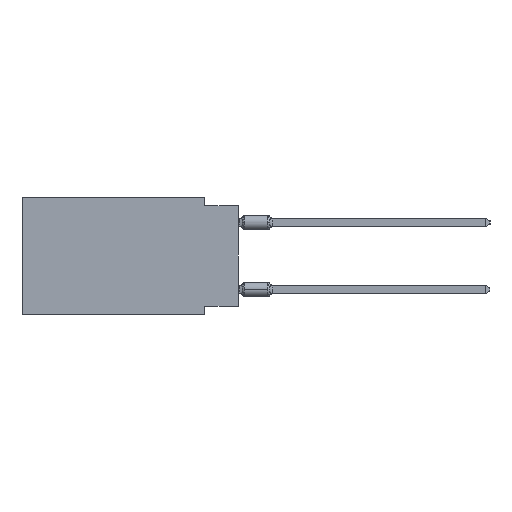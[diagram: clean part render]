
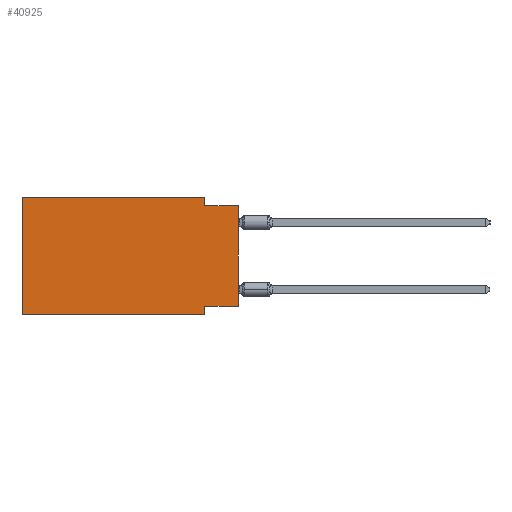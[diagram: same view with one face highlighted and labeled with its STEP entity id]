
A CAD part, left-side view. The second image highlights one B-rep face of the part: STEP entity #40925.
In plain terms, the highlighted planar face has unit normal (-1, 0, 0).
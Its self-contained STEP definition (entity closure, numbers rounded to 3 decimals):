
#448 = CARTESIAN_POINT ( 'NONE',  ( 0., 2.54, 0. ) ) ;
#1069 = VERTEX_POINT ( 'NONE', #16602 ) ;
#1219 = FACE_OUTER_BOUND ( 'NONE', #28514, .T. ) ;
#2025 = ORIENTED_EDGE ( 'NONE', *, *, #58208, .F. ) ;
#2263 = VECTOR ( 'NONE', #45250, 1000. ) ;
#3773 = CARTESIAN_POINT ( 'NONE',  ( 0., 2.54, -8.255 ) ) ;
#6072 = DIRECTION ( 'NONE',  ( 0., 0., -1. ) ) ;
#8190 = EDGE_CURVE ( 'NONE', #1069, #47045, #20040, .T. ) ;
#9418 = ORIENTED_EDGE ( 'NONE', *, *, #8190, .T. ) ;
#11039 = DIRECTION ( 'NONE',  ( 0., -1., 0. ) ) ;
#12231 = DIRECTION ( 'NONE',  ( 0., 1., 0. ) ) ;
#12298 = VERTEX_POINT ( 'NONE', #34679 ) ;
#12515 = VECTOR ( 'NONE', #12231, 1000. ) ;
#12544 = DIRECTION ( 'NONE',  ( 0., -1., 0. ) ) ;
#15291 = CARTESIAN_POINT ( 'NONE',  ( 0., 16.383, -8.89 ) ) ;
#15365 = VERTEX_POINT ( 'NONE', #53894 ) ;
#15708 = LINE ( 'NONE', #55323, #2263 ) ;
#16602 = CARTESIAN_POINT ( 'NONE',  ( 0., 0., -8.255 ) ) ;
#17701 = EDGE_CURVE ( 'NONE', #12298, #33344, #37183, .T. ) ;
#17742 = LINE ( 'NONE', #42714, #12515 ) ;
#17853 = VECTOR ( 'NONE', #39178, 1000. ) ;
#19060 = LINE ( 'NONE', #32686, #24188 ) ;
#19545 = VECTOR ( 'NONE', #12544, 1000. ) ;
#19724 = VERTEX_POINT ( 'NONE', #61601 ) ;
#20040 = LINE ( 'NONE', #44053, #17853 ) ;
#21690 = ORIENTED_EDGE ( 'NONE', *, *, #17701, .F. ) ;
#21887 = VERTEX_POINT ( 'NONE', #61754 ) ;
#24188 = VECTOR ( 'NONE', #29116, 1000. ) ;
#24577 = ORIENTED_EDGE ( 'NONE', *, *, #39522, .F. ) ;
#26257 = CARTESIAN_POINT ( 'NONE',  ( 0., 0., -0.635 ) ) ;
#27260 = ORIENTED_EDGE ( 'NONE', *, *, #46642, .F. ) ;
#28514 = EDGE_LOOP ( 'NONE', ( #9418, #2025, #44490, #21690, #63071, #38882, #27260, #24577 ) ) ;
#28870 = VECTOR ( 'NONE', #45242, 1000. ) ;
#29116 = DIRECTION ( 'NONE',  ( 0., -1., 0. ) ) ;
#31459 = EDGE_CURVE ( 'NONE', #21887, #15365, #49996, .T. ) ;
#32686 = CARTESIAN_POINT ( 'NONE',  ( 0., 0., -0.635 ) ) ;
#33344 = VERTEX_POINT ( 'NONE', #39706 ) ;
#34329 = DIRECTION ( 'NONE',  ( 1., 0., 0. ) ) ;
#34679 = CARTESIAN_POINT ( 'NONE',  ( 0., 16.383, 0. ) ) ;
#36195 = VERTEX_POINT ( 'NONE', #3773 ) ;
#37183 = LINE ( 'NONE', #57004, #19545 ) ;
#38882 = ORIENTED_EDGE ( 'NONE', *, *, #31459, .T. ) ;
#39178 = DIRECTION ( 'NONE',  ( 0., 0., 1. ) ) ;
#39522 = EDGE_CURVE ( 'NONE', #1069, #36195, #17742, .T. ) ;
#39706 = CARTESIAN_POINT ( 'NONE',  ( 0., 2.54, 0. ) ) ;
#39910 = VECTOR ( 'NONE', #11039, 1000. ) ;
#40925 = ADVANCED_FACE ( 'NONE', ( #1219 ), #50556, .F. ) ;
#41495 = VECTOR ( 'NONE', #61771, 1000. ) ;
#42714 = CARTESIAN_POINT ( 'NONE',  ( 0., 0., -8.255 ) ) ;
#44053 = CARTESIAN_POINT ( 'NONE',  ( 0., 0., 0. ) ) ;
#44490 = ORIENTED_EDGE ( 'NONE', *, *, #57133, .F. ) ;
#45242 = DIRECTION ( 'NONE',  ( 0., 0., -1. ) ) ;
#45250 = DIRECTION ( 'NONE',  ( 0., 0., 1. ) ) ;
#46642 = EDGE_CURVE ( 'NONE', #36195, #15365, #50112, .T. ) ;
#47002 = AXIS2_PLACEMENT_3D ( 'NONE', #59338, #34329, #6072 ) ;
#47045 = VERTEX_POINT ( 'NONE', #26257 ) ;
#49717 = EDGE_CURVE ( 'NONE', #21887, #12298, #15708, .T. ) ;
#49996 = LINE ( 'NONE', #15291, #39910 ) ;
#50112 = LINE ( 'NONE', #56579, #41495 ) ;
#50417 = LINE ( 'NONE', #448, #28870 ) ;
#50556 = PLANE ( 'NONE',  #47002 ) ;
#53894 = CARTESIAN_POINT ( 'NONE',  ( 0., 2.54, -8.89 ) ) ;
#55323 = CARTESIAN_POINT ( 'NONE',  ( 0., 16.383, 0. ) ) ;
#56579 = CARTESIAN_POINT ( 'NONE',  ( 0., 2.54, -8.89 ) ) ;
#57004 = CARTESIAN_POINT ( 'NONE',  ( 0., 16.383, 0. ) ) ;
#57133 = EDGE_CURVE ( 'NONE', #33344, #19724, #50417, .T. ) ;
#58208 = EDGE_CURVE ( 'NONE', #19724, #47045, #19060, .T. ) ;
#59338 = CARTESIAN_POINT ( 'NONE',  ( 0., 16.383, 0. ) ) ;
#61601 = CARTESIAN_POINT ( 'NONE',  ( 0., 2.54, -0.635 ) ) ;
#61754 = CARTESIAN_POINT ( 'NONE',  ( 0., 16.383, -8.89 ) ) ;
#61771 = DIRECTION ( 'NONE',  ( 0., 0., -1. ) ) ;
#63071 = ORIENTED_EDGE ( 'NONE', *, *, #49717, .F. ) ;
